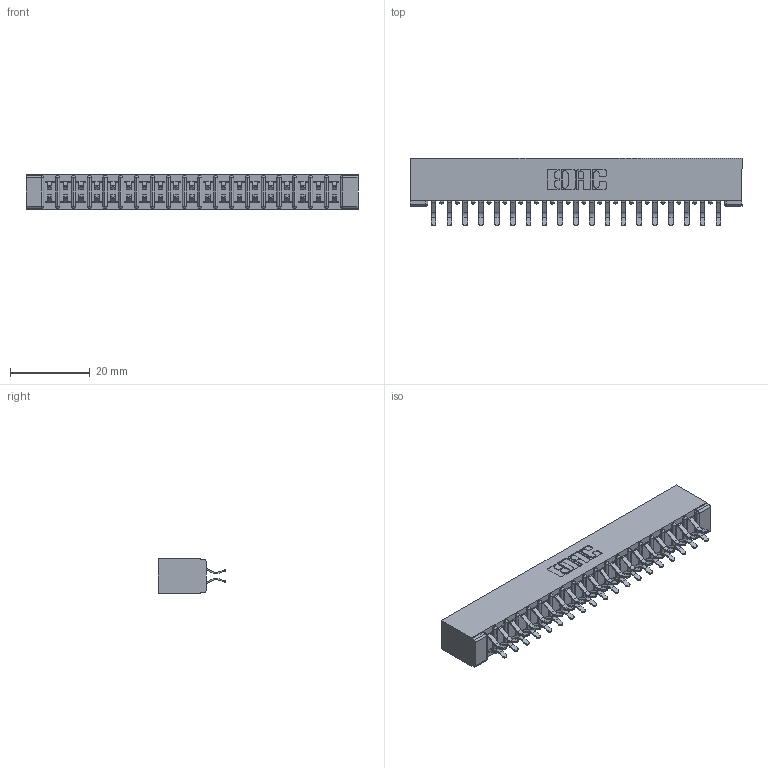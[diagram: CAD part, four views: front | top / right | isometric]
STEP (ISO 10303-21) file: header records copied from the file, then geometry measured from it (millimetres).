
FILE_DESCRIPTION (( 'STEP AP203' ), '1' );
FILE_NAME ('357-038-456-201.STEP', '2020-10-03T19:32:35', ( '' ), ( '' ), 'SwSTEP 2.0', 'SolidWorks 2020', '' );
FILE_SCHEMA (( 'CONFIG_CONTROL_DESIGN' ));
Length unit declared in the file: inch
Products named in the file (3): 307-290-001_556; 307 Part_No Mounting Lugs; 357-038-456-201
Assembly tree (39 placements, depth 2):
  357-038-456-201
    307 Part_No Mounting Lugs
    307-290-001_556  x38
Bounding box: 83.16 x 16.97 x 8.71 mm (x, y, z)
Volume: 5666.1 mm3; surface area: 10283.9 mm2
Topology: 39 solids, 39 shells, 2030 faces, 5695 edges, 3690 vertices
Faces by surface type: plane 1320, cylinder 670, sphere 40
Entity records: 19558 total; most frequent: CARTESIAN_POINT 3203, ORIENTED_EDGE 3170, DIRECTION 3147, EDGE_CURVE 1585, VECTOR 1207, LINE 1207, VERTEX_POINT 1026, AXIS2_PLACEMENT_3D 970
